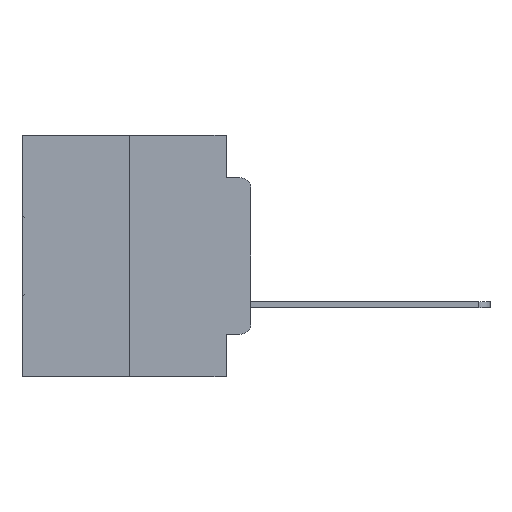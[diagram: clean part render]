
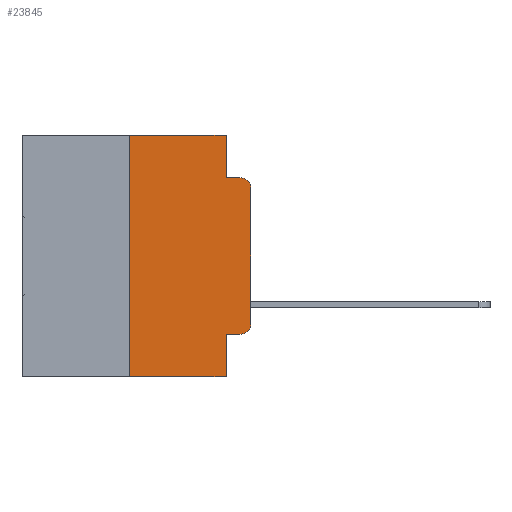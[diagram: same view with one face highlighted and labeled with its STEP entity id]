
A CAD part, left-side view. The second image highlights one B-rep face of the part: STEP entity #23845.
In plain terms, the highlighted planar face has unit normal (-1, 0, 0).
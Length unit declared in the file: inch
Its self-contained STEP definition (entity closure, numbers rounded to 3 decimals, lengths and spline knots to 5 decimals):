
#228 = FACE_OUTER_BOUND ( 'NONE', #6873, .T. ) ;
#232 = DIRECTION ( 'NONE',  ( 0., 0., 1. ) ) ;
#1088 = AXIS2_PLACEMENT_3D ( 'NONE', #24230, #9774, #26590 ) ;
#1282 = CARTESIAN_POINT ( 'NONE',  ( 0., 0.25, 0. ) ) ;
#1350 = VERTEX_POINT ( 'NONE', #5478 ) ;
#1536 = VERTEX_POINT ( 'NONE', #26805 ) ;
#1788 = CARTESIAN_POINT ( 'NONE',  ( 0., 0.02, -0.0885 ) ) ;
#2092 = CARTESIAN_POINT ( 'NONE',  ( 0., 0.02, -0.1085 ) ) ;
#2525 = ORIENTED_EDGE ( 'NONE', *, *, #13429, .F. ) ;
#2526 = DIRECTION ( 'NONE',  ( 0., 0., -1. ) ) ;
#2684 = VERTEX_POINT ( 'NONE', #1788 ) ;
#2907 = VERTEX_POINT ( 'NONE', #30718 ) ;
#3262 = VERTEX_POINT ( 'NONE', #30419 ) ;
#3550 = CARTESIAN_POINT ( 'NONE',  ( 0., 0.051, -0.0885 ) ) ;
#4683 = DIRECTION ( 'NONE',  ( 0., 0., -1. ) ) ;
#5478 = CARTESIAN_POINT ( 'NONE',  ( 0., 0.25, -0.5 ) ) ;
#6062 = VECTOR ( 'NONE', #29609, 39.37008 ) ;
#6132 = DIRECTION ( 'NONE',  ( 0., -1., 0. ) ) ;
#6873 = EDGE_LOOP ( 'NONE', ( #26259, #27846, #28360, #28864, #28921, #29651, #30626, #2525, #10185, #20796 ) ) ;
#6923 = DIRECTION ( 'NONE',  ( 0., -1., 0. ) ) ;
#7141 = EDGE_CURVE ( 'NONE', #1536, #3262, #11686, .T. ) ;
#7211 = CARTESIAN_POINT ( 'NONE',  ( 0., 0., -0.1085 ) ) ;
#7533 = LINE ( 'NONE', #1282, #23886 ) ;
#7869 = VERTEX_POINT ( 'NONE', #17432 ) ;
#8376 = AXIS2_PLACEMENT_3D ( 'NONE', #31539, #17553, #2526 ) ;
#9141 = CIRCLE ( 'NONE', #1088, 0.02 ) ;
#9774 = DIRECTION ( 'NONE',  ( -1., 0., 0. ) ) ;
#9973 = VERTEX_POINT ( 'NONE', #19921 ) ;
#10185 = ORIENTED_EDGE ( 'NONE', *, *, #7141, .T. ) ;
#10329 = VECTOR ( 'NONE', #6923, 39.37008 ) ;
#10527 = VECTOR ( 'NONE', #6132, 39.37008 ) ;
#10531 = CARTESIAN_POINT ( 'NONE',  ( 0., 0., 0. ) ) ;
#11502 = DIRECTION ( 'NONE',  ( 0., -1., 0. ) ) ;
#11603 = LINE ( 'NONE', #14409, #24396 ) ;
#11686 = LINE ( 'NONE', #28308, #28496 ) ;
#11931 = DIRECTION ( 'NONE',  ( 0., -1., 0. ) ) ;
#12772 = LINE ( 'NONE', #20174, #6062 ) ;
#13429 = EDGE_CURVE ( 'NONE', #1536, #7869, #12772, .T. ) ;
#14409 = CARTESIAN_POINT ( 'NONE',  ( 0., 0.473, -0.5 ) ) ;
#15436 = CARTESIAN_POINT ( 'NONE',  ( 0., 0., -0.3915 ) ) ;
#16125 = EDGE_CURVE ( 'NONE', #1350, #18271, #7533, .T. ) ;
#16554 = EDGE_CURVE ( 'NONE', #17756, #2684, #23857, .T. ) ;
#17432 = CARTESIAN_POINT ( 'NONE',  ( 0., 0.051, -0.5 ) ) ;
#17553 = DIRECTION ( 'NONE',  ( 1., 0., 0. ) ) ;
#17756 = VERTEX_POINT ( 'NONE', #7211 ) ;
#18271 = VERTEX_POINT ( 'NONE', #23114 ) ;
#19556 = DIRECTION ( 'NONE',  ( -1., 0., 0. ) ) ;
#19921 = CARTESIAN_POINT ( 'NONE',  ( 0., 0.051, 0. ) ) ;
#20174 = CARTESIAN_POINT ( 'NONE',  ( 0., 0.051, 0. ) ) ;
#20299 = AXIS2_PLACEMENT_3D ( 'NONE', #2092, #19556, #4683 ) ;
#20796 = ORIENTED_EDGE ( 'NONE', *, *, #28837, .T. ) ;
#21188 = LINE ( 'NONE', #24872, #26714 ) ;
#21237 = DIRECTION ( 'NONE',  ( 0., 0., 1. ) ) ;
#21639 = CARTESIAN_POINT ( 'NONE',  ( 0., 0.473, 0. ) ) ;
#22269 = VECTOR ( 'NONE', #232, 39.37008 ) ;
#23114 = CARTESIAN_POINT ( 'NONE',  ( 0., 0.25, 0. ) ) ;
#23160 = LINE ( 'NONE', #21639, #10329 ) ;
#23845 = ADVANCED_FACE ( 'NONE', ( #228 ), #29290, .F. ) ;
#23857 = CIRCLE ( 'NONE', #20299, 0.02 ) ;
#23886 = VECTOR ( 'NONE', #21237, 39.37008 ) ;
#24230 = CARTESIAN_POINT ( 'NONE',  ( 0., 0.02, -0.3915 ) ) ;
#24396 = VECTOR ( 'NONE', #11931, 39.37008 ) ;
#24872 = CARTESIAN_POINT ( 'NONE',  ( 0., 0.051, 0. ) ) ;
#24912 = EDGE_CURVE ( 'NONE', #9973, #2907, #21188, .T. ) ;
#25494 = EDGE_CURVE ( 'NONE', #29757, #17756, #28491, .T. ) ;
#25659 = EDGE_CURVE ( 'NONE', #2907, #2684, #29541, .T. ) ;
#26259 = ORIENTED_EDGE ( 'NONE', *, *, #25494, .T. ) ;
#26590 = DIRECTION ( 'NONE',  ( 0., 0., -1. ) ) ;
#26714 = VECTOR ( 'NONE', #29529, 39.37008 ) ;
#26805 = CARTESIAN_POINT ( 'NONE',  ( 0., 0.051, -0.4115 ) ) ;
#27846 = ORIENTED_EDGE ( 'NONE', *, *, #16554, .T. ) ;
#28308 = CARTESIAN_POINT ( 'NONE',  ( 0., 0.051, -0.4115 ) ) ;
#28360 = ORIENTED_EDGE ( 'NONE', *, *, #25659, .F. ) ;
#28491 = LINE ( 'NONE', #10531, #22269 ) ;
#28496 = VECTOR ( 'NONE', #11502, 39.37008 ) ;
#28837 = EDGE_CURVE ( 'NONE', #3262, #29757, #9141, .T. ) ;
#28864 = ORIENTED_EDGE ( 'NONE', *, *, #24912, .F. ) ;
#28921 = ORIENTED_EDGE ( 'NONE', *, *, #29451, .F. ) ;
#29290 = PLANE ( 'NONE',  #8376 ) ;
#29451 = EDGE_CURVE ( 'NONE', #18271, #9973, #23160, .T. ) ;
#29529 = DIRECTION ( 'NONE',  ( 0., 0., -1. ) ) ;
#29541 = LINE ( 'NONE', #3550, #10527 ) ;
#29609 = DIRECTION ( 'NONE',  ( 0., 0., -1. ) ) ;
#29651 = ORIENTED_EDGE ( 'NONE', *, *, #16125, .F. ) ;
#29757 = VERTEX_POINT ( 'NONE', #15436 ) ;
#30419 = CARTESIAN_POINT ( 'NONE',  ( 0., 0.02, -0.4115 ) ) ;
#30626 = ORIENTED_EDGE ( 'NONE', *, *, #31240, .T. ) ;
#30718 = CARTESIAN_POINT ( 'NONE',  ( 0., 0.051, -0.0885 ) ) ;
#31240 = EDGE_CURVE ( 'NONE', #1350, #7869, #11603, .T. ) ;
#31539 = CARTESIAN_POINT ( 'NONE',  ( 0., 0.473, 0. ) ) ;
